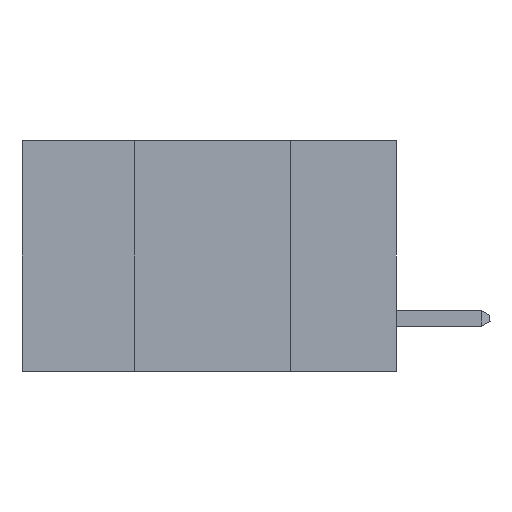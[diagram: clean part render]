
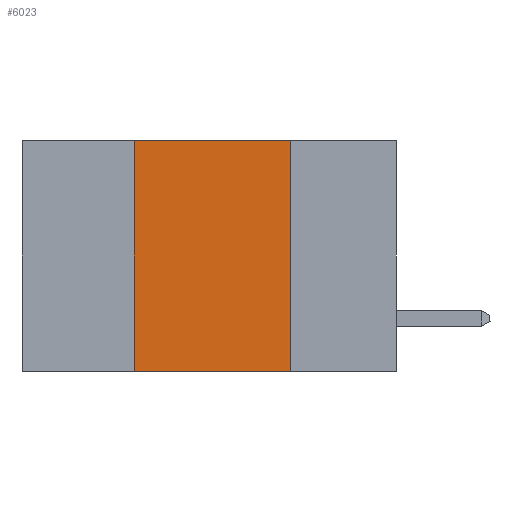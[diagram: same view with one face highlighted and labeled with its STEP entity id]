
A CAD part, left-side view. The second image highlights one B-rep face of the part: STEP entity #6023.
In plain terms, the highlighted planar face has unit normal (-1, 0, 0).
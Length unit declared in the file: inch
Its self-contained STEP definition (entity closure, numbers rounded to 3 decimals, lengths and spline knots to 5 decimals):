
#11 = ORIENTED_EDGE ( 'NONE', *, *, #5339, .F. ) ;
#12 = CARTESIAN_POINT ( 'NONE',  ( 0., 0.17, -0.37 ) ) ;
#46 = ORIENTED_EDGE ( 'NONE', *, *, #7116, .F. ) ;
#215 = VERTEX_POINT ( 'NONE', #12 ) ;
#226 = ORIENTED_EDGE ( 'NONE', *, *, #5701, .T. ) ;
#275 = ORIENTED_EDGE ( 'NONE', *, *, #7577, .F. ) ;
#376 = VECTOR ( 'NONE', #9828, 39.37008 ) ;
#757 = AXIS2_PLACEMENT_3D ( 'NONE', #3039, #4835, #3105 ) ;
#1325 = CARTESIAN_POINT ( 'NONE',  ( 0., 0.6, -0.37 ) ) ;
#1971 = VERTEX_POINT ( 'NONE', #7598 ) ;
#2631 = LINE ( 'NONE', #1325, #376 ) ;
#3006 = VECTOR ( 'NONE', #9132, 39.37008 ) ;
#3039 = CARTESIAN_POINT ( 'NONE',  ( 0., 0.6, 0. ) ) ;
#3105 = DIRECTION ( 'NONE',  ( 0., 0., -1. ) ) ;
#3653 = VERTEX_POINT ( 'NONE', #9279 ) ;
#3655 = DIRECTION ( 'NONE',  ( 0., 0., -1. ) ) ;
#3813 = PLANE ( 'NONE',  #757 ) ;
#4793 = EDGE_LOOP ( 'NONE', ( #46, #275, #11, #226 ) ) ;
#4835 = DIRECTION ( 'NONE',  ( 1., 0., 0. ) ) ;
#5015 = VERTEX_POINT ( 'NONE', #6048 ) ;
#5130 = VECTOR ( 'NONE', #3655, 39.37008 ) ;
#5331 = LINE ( 'NONE', #6049, #7320 ) ;
#5339 = EDGE_CURVE ( 'NONE', #3653, #1971, #5331, .T. ) ;
#5701 = EDGE_CURVE ( 'NONE', #3653, #215, #2631, .T. ) ;
#6023 = ADVANCED_FACE ( 'NONE', ( #8814 ), #3813, .F. ) ;
#6048 = CARTESIAN_POINT ( 'NONE',  ( 0., 0.17, 0. ) ) ;
#6049 = CARTESIAN_POINT ( 'NONE',  ( 0., 0.42, 0. ) ) ;
#6291 = CARTESIAN_POINT ( 'NONE',  ( 0., 0.17, 0. ) ) ;
#7019 = DIRECTION ( 'NONE',  ( 0., 0., 1. ) ) ;
#7116 = EDGE_CURVE ( 'NONE', #5015, #215, #9479, .T. ) ;
#7320 = VECTOR ( 'NONE', #7019, 39.37008 ) ;
#7577 = EDGE_CURVE ( 'NONE', #1971, #5015, #9229, .T. ) ;
#7598 = CARTESIAN_POINT ( 'NONE',  ( 0., 0.42, 0. ) ) ;
#8477 = CARTESIAN_POINT ( 'NONE',  ( 0., 0.6, 0. ) ) ;
#8814 = FACE_OUTER_BOUND ( 'NONE', #4793, .T. ) ;
#9132 = DIRECTION ( 'NONE',  ( 0., -1., 0. ) ) ;
#9229 = LINE ( 'NONE', #8477, #3006 ) ;
#9279 = CARTESIAN_POINT ( 'NONE',  ( 0., 0.42, -0.37 ) ) ;
#9479 = LINE ( 'NONE', #6291, #5130 ) ;
#9828 = DIRECTION ( 'NONE',  ( 0., -1., 0. ) ) ;
